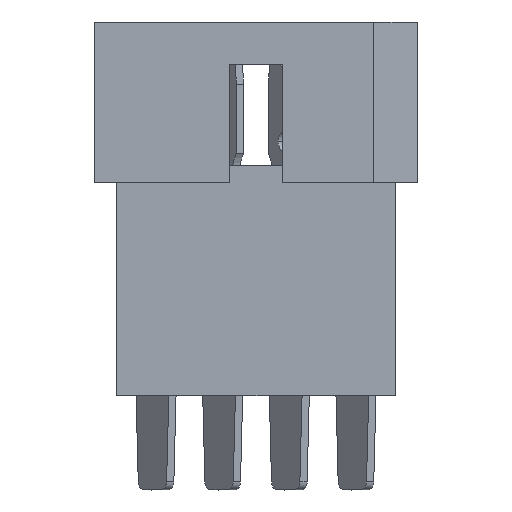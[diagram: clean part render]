
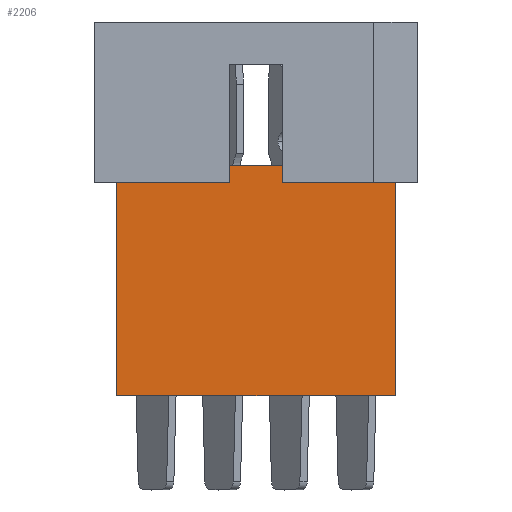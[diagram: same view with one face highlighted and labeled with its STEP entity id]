
A CAD part, top view. The second image highlights one B-rep face of the part: STEP entity #2206.
In plain terms, the highlighted planar face has unit normal (0, 0, 1).
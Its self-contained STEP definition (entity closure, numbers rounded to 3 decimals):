
#18 = CARTESIAN_POINT ( 'NONE',  ( -2.324, -12.7, 2.54 ) ) ;
#63 = VECTOR ( 'NONE', #3446, 1000. ) ;
#69 = CARTESIAN_POINT ( 'NONE',  ( -2.324, -12.7, 2.54 ) ) ;
#135 = EDGE_CURVE ( 'NONE', #7089, #4947, #258, .T. ) ;
#157 = CARTESIAN_POINT ( 'NONE',  ( 4.343, 1.016, 2.54 ) ) ;
#258 = LINE ( 'NONE', #4410, #3571 ) ;
#339 = EDGE_CURVE ( 'NONE', #3274, #5009, #2474, .T. ) ;
#367 = LINE ( 'NONE', #5563, #7259 ) ;
#413 = EDGE_CURVE ( 'NONE', #7089, #2108, #4819, .T. ) ;
#425 = VECTOR ( 'NONE', #6793, 1000. ) ;
#613 = CARTESIAN_POINT ( 'NONE',  ( 0., 1.016, 2.54 ) ) ;
#735 = ORIENTED_EDGE ( 'NONE', *, *, #3904, .F. ) ;
#1010 = CARTESIAN_POINT ( 'NONE',  ( -2.324, -12.7, 2.54 ) ) ;
#1677 = DIRECTION ( 'NONE',  ( 0., 1., 0. ) ) ;
#1979 = ORIENTED_EDGE ( 'NONE', *, *, #2141, .T. ) ;
#2108 = VERTEX_POINT ( 'NONE', #3691 ) ;
#2141 = EDGE_CURVE ( 'NONE', #6261, #3274, #6133, .T. ) ;
#2146 = ORIENTED_EDGE ( 'NONE', *, *, #339, .T. ) ;
#2206 = ADVANCED_FACE ( 'NONE', ( #4623 ), #2599, .T. ) ;
#2474 = LINE ( 'NONE', #3425, #425 ) ;
#2532 = CARTESIAN_POINT ( 'NONE',  ( -2.324, 0., 2.54 ) ) ;
#2599 = PLANE ( 'NONE',  #4225 ) ;
#2874 = VECTOR ( 'NONE', #3544, 1000. ) ;
#3213 = ORIENTED_EDGE ( 'NONE', *, *, #135, .T. ) ;
#3223 = DIRECTION ( 'NONE',  ( 0., 0., 1. ) ) ;
#3274 = VERTEX_POINT ( 'NONE', #4363 ) ;
#3425 = CARTESIAN_POINT ( 'NONE',  ( 14.211, -12.7, 2.54 ) ) ;
#3446 = DIRECTION ( 'NONE',  ( 1., 0., 0. ) ) ;
#3544 = DIRECTION ( 'NONE',  ( 1., 0., 0. ) ) ;
#3571 = VECTOR ( 'NONE', #6751, 1000. ) ;
#3667 = DIRECTION ( 'NONE',  ( 1., 0., 0. ) ) ;
#3691 = CARTESIAN_POINT ( 'NONE',  ( 7.544, 1.016, 2.54 ) ) ;
#3904 = EDGE_CURVE ( 'NONE', #6547, #5009, #6568, .T. ) ;
#3976 = CARTESIAN_POINT ( 'NONE',  ( 14.211, 0., 2.54 ) ) ;
#4087 = ORIENTED_EDGE ( 'NONE', *, *, #6171, .F. ) ;
#4125 = LINE ( 'NONE', #69, #4668 ) ;
#4185 = DIRECTION ( 'NONE',  ( 0., 1., 0. ) ) ;
#4225 = AXIS2_PLACEMENT_3D ( 'NONE', #1010, #3223, #5012 ) ;
#4363 = CARTESIAN_POINT ( 'NONE',  ( 14.211, -12.7, 2.54 ) ) ;
#4410 = CARTESIAN_POINT ( 'NONE',  ( 4.343, 6.985, 2.54 ) ) ;
#4426 = EDGE_CURVE ( 'NONE', #6547, #2108, #367, .T. ) ;
#4543 = LINE ( 'NONE', #7300, #63 ) ;
#4578 = ORIENTED_EDGE ( 'NONE', *, *, #413, .F. ) ;
#4621 = DIRECTION ( 'NONE',  ( 1., 0., 0. ) ) ;
#4623 = FACE_OUTER_BOUND ( 'NONE', #4804, .T. ) ;
#4668 = VECTOR ( 'NONE', #4185, 1000. ) ;
#4804 = EDGE_LOOP ( 'NONE', ( #4087, #7231, #1979, #2146, #735, #7237, #4578, #3213 ) ) ;
#4819 = LINE ( 'NONE', #613, #7070 ) ;
#4947 = VERTEX_POINT ( 'NONE', #6230 ) ;
#5009 = VERTEX_POINT ( 'NONE', #3976 ) ;
#5012 = DIRECTION ( 'NONE',  ( 1., 0., 0. ) ) ;
#5121 = EDGE_CURVE ( 'NONE', #6261, #6546, #4125, .T. ) ;
#5475 = CARTESIAN_POINT ( 'NONE',  ( -2.324, -12.7, 2.54 ) ) ;
#5517 = VECTOR ( 'NONE', #3667, 1000. ) ;
#5563 = CARTESIAN_POINT ( 'NONE',  ( 7.544, 6.985, 2.54 ) ) ;
#6133 = LINE ( 'NONE', #5475, #5517 ) ;
#6171 = EDGE_CURVE ( 'NONE', #6546, #4947, #4543, .T. ) ;
#6230 = CARTESIAN_POINT ( 'NONE',  ( 4.343, 0., 2.54 ) ) ;
#6261 = VERTEX_POINT ( 'NONE', #18 ) ;
#6521 = CARTESIAN_POINT ( 'NONE',  ( 7.544, 0., 2.54 ) ) ;
#6546 = VERTEX_POINT ( 'NONE', #2532 ) ;
#6547 = VERTEX_POINT ( 'NONE', #6521 ) ;
#6568 = LINE ( 'NONE', #6936, #2874 ) ;
#6751 = DIRECTION ( 'NONE',  ( 0., -1., 0. ) ) ;
#6793 = DIRECTION ( 'NONE',  ( 0., 1., 0. ) ) ;
#6936 = CARTESIAN_POINT ( 'NONE',  ( -2.324, 0., 2.54 ) ) ;
#7070 = VECTOR ( 'NONE', #4621, 1000. ) ;
#7089 = VERTEX_POINT ( 'NONE', #157 ) ;
#7231 = ORIENTED_EDGE ( 'NONE', *, *, #5121, .F. ) ;
#7237 = ORIENTED_EDGE ( 'NONE', *, *, #4426, .T. ) ;
#7259 = VECTOR ( 'NONE', #1677, 1000. ) ;
#7300 = CARTESIAN_POINT ( 'NONE',  ( -2.324, 0., 2.54 ) ) ;
